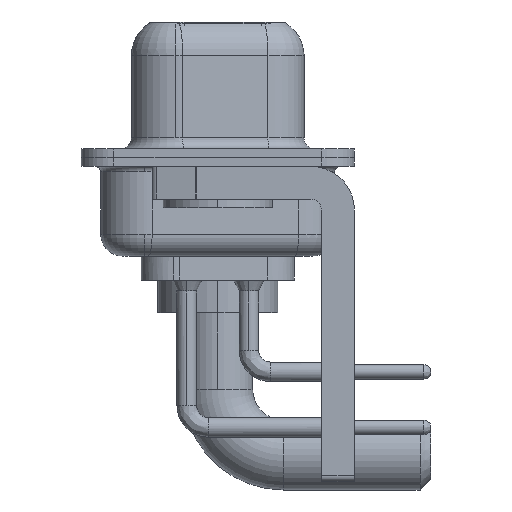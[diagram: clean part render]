
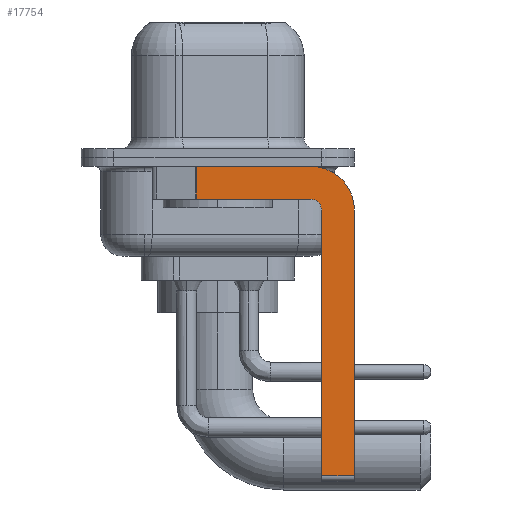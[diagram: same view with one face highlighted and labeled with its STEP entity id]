
A CAD part, left-side view. The second image highlights one B-rep face of the part: STEP entity #17754.
In plain terms, the highlighted planar face has unit normal (-1, 0, 0).
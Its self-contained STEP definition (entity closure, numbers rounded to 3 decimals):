
#62 = VECTOR ( 'NONE', #4009, 1000. ) ;
#75 = AXIS2_PLACEMENT_3D ( 'NONE', #8999, #1615, #7327 ) ;
#277 = DIRECTION ( 'NONE',  ( 0., 0., -1. ) ) ;
#856 = ORIENTED_EDGE ( 'NONE', *, *, #12670, .F. ) ;
#1173 = LINE ( 'NONE', #17593, #8834 ) ;
#1513 = EDGE_LOOP ( 'NONE', ( #12062, #2181, #18642, #6483, #7251, #9157, #856, #19141 ) ) ;
#1534 = VERTEX_POINT ( 'NONE', #16628 ) ;
#1615 = DIRECTION ( 'NONE',  ( -1., 0., 0. ) ) ;
#1763 = AXIS2_PLACEMENT_3D ( 'NONE', #6184, #13848, #277 ) ;
#2181 = ORIENTED_EDGE ( 'NONE', *, *, #6473, .T. ) ;
#2445 = CARTESIAN_POINT ( 'NONE',  ( -2.9, 0.978, -1.9 ) ) ;
#2905 = LINE ( 'NONE', #13409, #9008 ) ;
#2926 = CARTESIAN_POINT ( 'NONE',  ( -2.9, -6.25, -2.4 ) ) ;
#3369 = CARTESIAN_POINT ( 'NONE',  ( -2.9, -6.25, -14.55 ) ) ;
#4009 = DIRECTION ( 'NONE',  ( 0., 0., 1. ) ) ;
#4616 = VERTEX_POINT ( 'NONE', #8549 ) ;
#5323 = CARTESIAN_POINT ( 'NONE',  ( -2.9, 3., -0.4 ) ) ;
#5663 = DIRECTION ( 'NONE',  ( 0., 0., -1. ) ) ;
#5895 = EDGE_CURVE ( 'NONE', #4616, #14939, #1173, .T. ) ;
#6157 = CIRCLE ( 'NONE', #1763, 2. ) ;
#6184 = CARTESIAN_POINT ( 'NONE',  ( -2.9, -4.25, -2.4 ) ) ;
#6473 = EDGE_CURVE ( 'NONE', #10053, #14939, #19139, .T. ) ;
#6483 = ORIENTED_EDGE ( 'NONE', *, *, #18620, .F. ) ;
#6878 = DIRECTION ( 'NONE',  ( 0., 0., -1. ) ) ;
#7251 = ORIENTED_EDGE ( 'NONE', *, *, #17008, .F. ) ;
#7327 = DIRECTION ( 'NONE',  ( 0., 0., 1. ) ) ;
#7755 = CARTESIAN_POINT ( 'NONE',  ( -2.9, -4.75, -2.4 ) ) ;
#7871 = VERTEX_POINT ( 'NONE', #8912 ) ;
#8546 = CARTESIAN_POINT ( 'NONE',  ( -2.9, -4.25, -2.4 ) ) ;
#8549 = CARTESIAN_POINT ( 'NONE',  ( -2.9, -4.25, -1.9 ) ) ;
#8759 = LINE ( 'NONE', #5323, #16055 ) ;
#8834 = VECTOR ( 'NONE', #16116, 1000. ) ;
#8904 = DIRECTION ( 'NONE',  ( 0., 0., -1. ) ) ;
#8912 = CARTESIAN_POINT ( 'NONE',  ( -2.9, -4.75, -14.55 ) ) ;
#8999 = CARTESIAN_POINT ( 'NONE',  ( -2.9, -4.25, -2.4 ) ) ;
#9008 = VECTOR ( 'NONE', #8904, 1000. ) ;
#9157 = ORIENTED_EDGE ( 'NONE', *, *, #16711, .T. ) ;
#10053 = VERTEX_POINT ( 'NONE', #16317 ) ;
#10298 = CARTESIAN_POINT ( 'NONE',  ( -2.9, -4.25, -14.55 ) ) ;
#10609 = CARTESIAN_POINT ( 'NONE',  ( -2.9, 0.978, -1.9 ) ) ;
#10948 = VERTEX_POINT ( 'NONE', #2926 ) ;
#11319 = DIRECTION ( 'NONE',  ( 0., -1., 0. ) ) ;
#11382 = CIRCLE ( 'NONE', #75, 0.5 ) ;
#11397 = FACE_OUTER_BOUND ( 'NONE', #1513, .T. ) ;
#11926 = EDGE_CURVE ( 'NONE', #1534, #10948, #6157, .T. ) ;
#11985 = VECTOR ( 'NONE', #16292, 1000. ) ;
#12022 = VERTEX_POINT ( 'NONE', #7755 ) ;
#12062 = ORIENTED_EDGE ( 'NONE', *, *, #16091, .F. ) ;
#12071 = LINE ( 'NONE', #10298, #11985 ) ;
#12670 = EDGE_CURVE ( 'NONE', #10948, #19273, #2905, .T. ) ;
#13251 = VECTOR ( 'NONE', #5663, 1000. ) ;
#13409 = CARTESIAN_POINT ( 'NONE',  ( -2.9, -6.25, -2.4 ) ) ;
#13848 = DIRECTION ( 'NONE',  ( 1., 0., 0. ) ) ;
#14188 = AXIS2_PLACEMENT_3D ( 'NONE', #8546, #19155, #6878 ) ;
#14445 = PLANE ( 'NONE',  #14188 ) ;
#14939 = VERTEX_POINT ( 'NONE', #10609 ) ;
#16055 = VECTOR ( 'NONE', #11319, 1000. ) ;
#16091 = EDGE_CURVE ( 'NONE', #10053, #1534, #8759, .T. ) ;
#16116 = DIRECTION ( 'NONE',  ( 0., 1., 0. ) ) ;
#16292 = DIRECTION ( 'NONE',  ( 0., -1., 0. ) ) ;
#16317 = CARTESIAN_POINT ( 'NONE',  ( -2.9, 0.978, -0.4 ) ) ;
#16628 = CARTESIAN_POINT ( 'NONE',  ( -2.9, -4.25, -0.4 ) ) ;
#16711 = EDGE_CURVE ( 'NONE', #7871, #19273, #12071, .T. ) ;
#17008 = EDGE_CURVE ( 'NONE', #7871, #12022, #18846, .T. ) ;
#17593 = CARTESIAN_POINT ( 'NONE',  ( -2.9, -4.25, -1.9 ) ) ;
#17754 = ADVANCED_FACE ( 'NONE', ( #11397 ), #14445, .F. ) ;
#18620 = EDGE_CURVE ( 'NONE', #12022, #4616, #11382, .T. ) ;
#18642 = ORIENTED_EDGE ( 'NONE', *, *, #5895, .F. ) ;
#18846 = LINE ( 'NONE', #19133, #62 ) ;
#19133 = CARTESIAN_POINT ( 'NONE',  ( -2.9, -4.75, -14.8 ) ) ;
#19139 = LINE ( 'NONE', #2445, #13251 ) ;
#19141 = ORIENTED_EDGE ( 'NONE', *, *, #11926, .F. ) ;
#19155 = DIRECTION ( 'NONE',  ( 1., 0., 0. ) ) ;
#19273 = VERTEX_POINT ( 'NONE', #3369 ) ;
